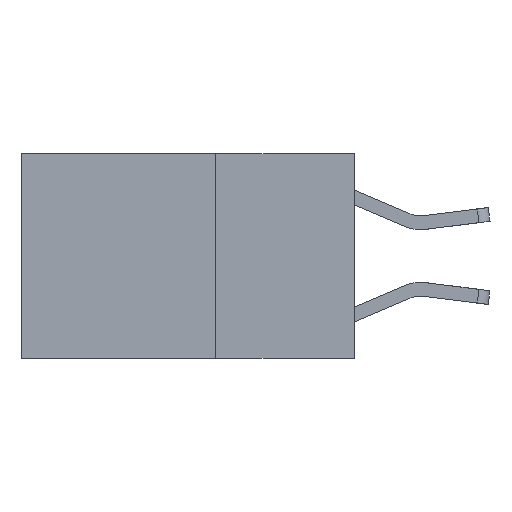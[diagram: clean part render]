
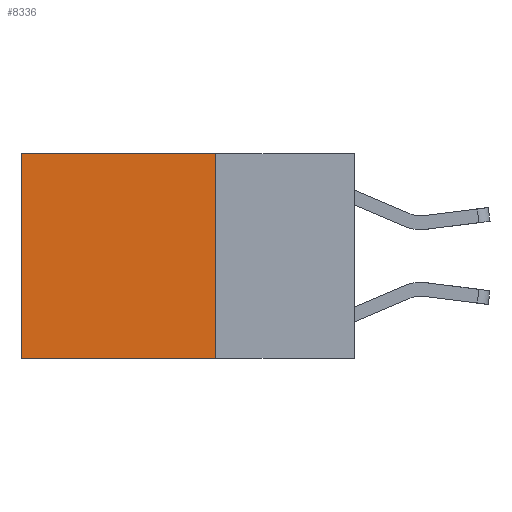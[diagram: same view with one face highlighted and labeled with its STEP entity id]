
A CAD part, left-side view. The second image highlights one B-rep face of the part: STEP entity #8336.
In plain terms, the highlighted planar face has unit normal (-1, 0, 0).
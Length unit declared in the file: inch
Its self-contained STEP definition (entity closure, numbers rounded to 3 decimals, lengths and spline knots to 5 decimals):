
#857 = EDGE_LOOP ( 'NONE', ( #5199, #4930, #5611, #8339 ) ) ;
#885 = LINE ( 'NONE', #9026, #5085 ) ;
#1414 = VERTEX_POINT ( 'NONE', #5044 ) ;
#2102 = AXIS2_PLACEMENT_3D ( 'NONE', #7620, #2620, #8432 ) ;
#2295 = VECTOR ( 'NONE', #8979, 39.37008 ) ;
#2620 = DIRECTION ( 'NONE',  ( 1., 0., 0. ) ) ;
#3994 = VERTEX_POINT ( 'NONE', #8375 ) ;
#4670 = DIRECTION ( 'NONE',  ( 0., 1., 0. ) ) ;
#4930 = ORIENTED_EDGE ( 'NONE', *, *, #5152, .F. ) ;
#5031 = EDGE_CURVE ( 'NONE', #5281, #1414, #5921, .T. ) ;
#5044 = CARTESIAN_POINT ( 'NONE',  ( 0.2625, 0.6, -0.37 ) ) ;
#5085 = VECTOR ( 'NONE', #9801, 39.37008 ) ;
#5152 = EDGE_CURVE ( 'NONE', #3994, #1414, #8876, .T. ) ;
#5199 = ORIENTED_EDGE ( 'NONE', *, *, #5031, .T. ) ;
#5281 = VERTEX_POINT ( 'NONE', #9172 ) ;
#5362 = LINE ( 'NONE', #6386, #7491 ) ;
#5611 = ORIENTED_EDGE ( 'NONE', *, *, #10407, .F. ) ;
#5921 = LINE ( 'NONE', #9596, #10056 ) ;
#6386 = CARTESIAN_POINT ( 'NONE',  ( 0.2625, 0.25, 0. ) ) ;
#6396 = EDGE_CURVE ( 'NONE', #7816, #5281, #5362, .T. ) ;
#6632 = CARTESIAN_POINT ( 'NONE',  ( 0.2625, 0.25, -0.37 ) ) ;
#7491 = VECTOR ( 'NONE', #4670, 39.37008 ) ;
#7620 = CARTESIAN_POINT ( 'NONE',  ( 0.2625, 0.25, 0. ) ) ;
#7816 = VERTEX_POINT ( 'NONE', #10102 ) ;
#8336 = ADVANCED_FACE ( 'NONE', ( #9905 ), #9921, .F. ) ;
#8339 = ORIENTED_EDGE ( 'NONE', *, *, #6396, .T. ) ;
#8375 = CARTESIAN_POINT ( 'NONE',  ( 0.2625, 0.25, -0.37 ) ) ;
#8432 = DIRECTION ( 'NONE',  ( 0., 0., -1. ) ) ;
#8876 = LINE ( 'NONE', #6632, #2295 ) ;
#8979 = DIRECTION ( 'NONE',  ( 0., 1., 0. ) ) ;
#9026 = CARTESIAN_POINT ( 'NONE',  ( 0.2625, 0.25, 0. ) ) ;
#9172 = CARTESIAN_POINT ( 'NONE',  ( 0.2625, 0.6, 0. ) ) ;
#9596 = CARTESIAN_POINT ( 'NONE',  ( 0.2625, 0.6, 0. ) ) ;
#9801 = DIRECTION ( 'NONE',  ( 0., 0., -1. ) ) ;
#9905 = FACE_OUTER_BOUND ( 'NONE', #857, .T. ) ;
#9921 = PLANE ( 'NONE',  #2102 ) ;
#10056 = VECTOR ( 'NONE', #10335, 39.37008 ) ;
#10102 = CARTESIAN_POINT ( 'NONE',  ( 0.2625, 0.25, 0. ) ) ;
#10335 = DIRECTION ( 'NONE',  ( 0., 0., -1. ) ) ;
#10407 = EDGE_CURVE ( 'NONE', #7816, #3994, #885, .T. ) ;
